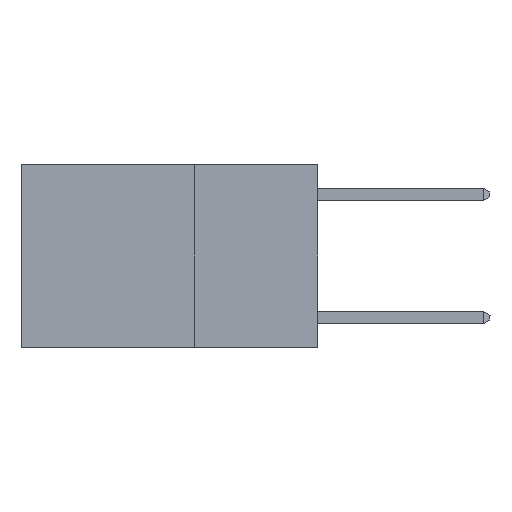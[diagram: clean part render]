
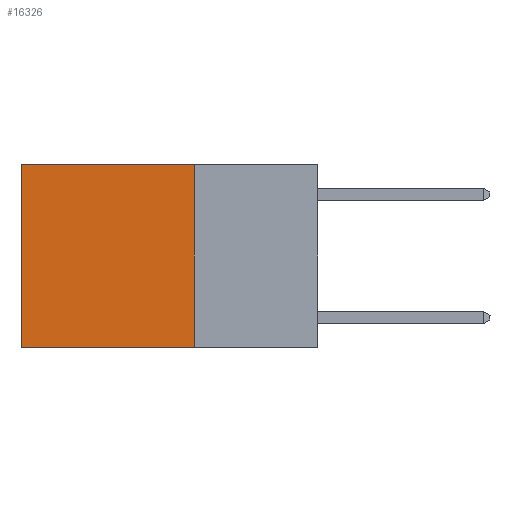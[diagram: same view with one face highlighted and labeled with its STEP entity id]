
A CAD part, left-side view. The second image highlights one B-rep face of the part: STEP entity #16326.
In plain terms, the highlighted planar face has unit normal (-1, 0, 0).
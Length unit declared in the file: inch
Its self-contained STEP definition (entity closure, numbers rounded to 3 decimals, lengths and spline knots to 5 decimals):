
#470 = VERTEX_POINT ( 'NONE', #14481 ) ;
#1136 = CARTESIAN_POINT ( 'NONE',  ( 0.2625, 0.25, -0.37 ) ) ;
#1502 = ORIENTED_EDGE ( 'NONE', *, *, #15273, .F. ) ;
#1616 = CARTESIAN_POINT ( 'NONE',  ( 0.2625, 0.25, 0. ) ) ;
#3862 = CARTESIAN_POINT ( 'NONE',  ( 0.2625, 0.6, 0. ) ) ;
#4161 = LINE ( 'NONE', #1136, #11441 ) ;
#4387 = EDGE_LOOP ( 'NONE', ( #15580, #11989, #1502, #17800 ) ) ;
#4546 = DIRECTION ( 'NONE',  ( 0., 0., -1. ) ) ;
#4614 = VECTOR ( 'NONE', #6198, 39.37008 ) ;
#5631 = DIRECTION ( 'NONE',  ( 0., 0., -1. ) ) ;
#6198 = DIRECTION ( 'NONE',  ( 0., 1., 0. ) ) ;
#6269 = CARTESIAN_POINT ( 'NONE',  ( 0.2625, 0.6, -0.37 ) ) ;
#8219 = DIRECTION ( 'NONE',  ( 0., 0., -1. ) ) ;
#8220 = DIRECTION ( 'NONE',  ( 0., 1., 0. ) ) ;
#8516 = VECTOR ( 'NONE', #8219, 39.37008 ) ;
#9498 = LINE ( 'NONE', #1616, #8516 ) ;
#9849 = CARTESIAN_POINT ( 'NONE',  ( 0.2625, 0.25, -0.37 ) ) ;
#10614 = CARTESIAN_POINT ( 'NONE',  ( 0.2625, 0.6, 0. ) ) ;
#11441 = VECTOR ( 'NONE', #8220, 39.37008 ) ;
#11929 = LINE ( 'NONE', #10614, #15394 ) ;
#11989 = ORIENTED_EDGE ( 'NONE', *, *, #15699, .F. ) ;
#12457 = PLANE ( 'NONE',  #15946 ) ;
#12633 = LINE ( 'NONE', #14146, #4614 ) ;
#13723 = EDGE_CURVE ( 'NONE', #470, #20272, #12633, .T. ) ;
#14146 = CARTESIAN_POINT ( 'NONE',  ( 0.2625, 0.25, 0. ) ) ;
#14481 = CARTESIAN_POINT ( 'NONE',  ( 0.2625, 0.25, 0. ) ) ;
#15273 = EDGE_CURVE ( 'NONE', #470, #16908, #9498, .T. ) ;
#15394 = VECTOR ( 'NONE', #5631, 39.37008 ) ;
#15509 = EDGE_CURVE ( 'NONE', #20272, #19680, #11929, .T. ) ;
#15580 = ORIENTED_EDGE ( 'NONE', *, *, #15509, .T. ) ;
#15699 = EDGE_CURVE ( 'NONE', #16908, #19680, #4161, .T. ) ;
#15730 = CARTESIAN_POINT ( 'NONE',  ( 0.2625, 0.25, 0. ) ) ;
#15936 = DIRECTION ( 'NONE',  ( 1., 0., 0. ) ) ;
#15946 = AXIS2_PLACEMENT_3D ( 'NONE', #15730, #15936, #4546 ) ;
#16326 = ADVANCED_FACE ( 'NONE', ( #18660 ), #12457, .F. ) ;
#16908 = VERTEX_POINT ( 'NONE', #9849 ) ;
#17800 = ORIENTED_EDGE ( 'NONE', *, *, #13723, .T. ) ;
#18660 = FACE_OUTER_BOUND ( 'NONE', #4387, .T. ) ;
#19680 = VERTEX_POINT ( 'NONE', #6269 ) ;
#20272 = VERTEX_POINT ( 'NONE', #3862 ) ;
